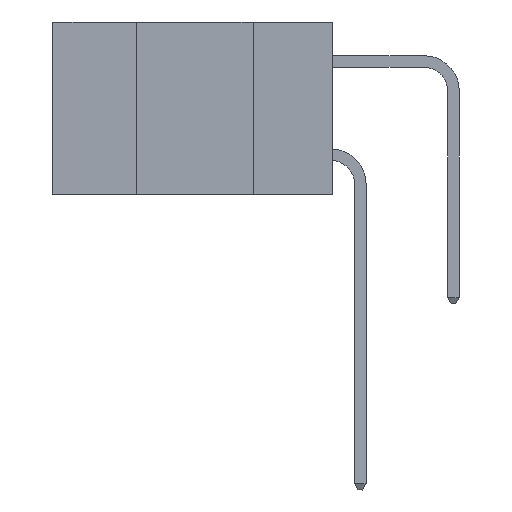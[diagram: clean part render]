
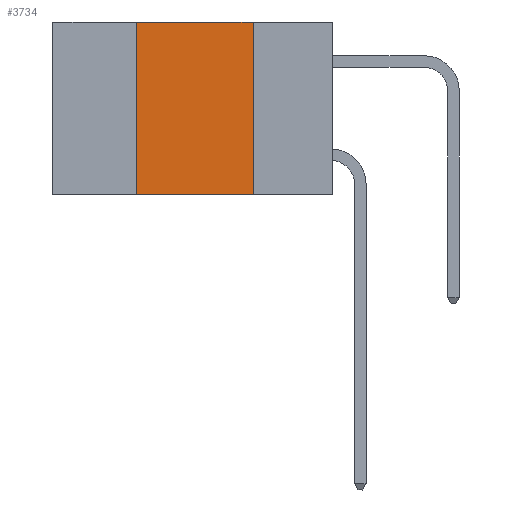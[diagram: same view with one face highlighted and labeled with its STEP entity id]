
A CAD part, left-side view. The second image highlights one B-rep face of the part: STEP entity #3734.
In plain terms, the highlighted planar face has unit normal (-1, 0, 0).
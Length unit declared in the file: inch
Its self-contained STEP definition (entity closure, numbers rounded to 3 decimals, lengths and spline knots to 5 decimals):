
#967 = EDGE_LOOP ( 'NONE', ( #6761, #6715, #1162, #23691 ) ) ;
#1009 = EDGE_CURVE ( 'NONE', #8339, #14403, #14055, .T. ) ;
#1162 = ORIENTED_EDGE ( 'NONE', *, *, #10354, .F. ) ;
#1880 = VERTEX_POINT ( 'NONE', #25369 ) ;
#2303 = FACE_OUTER_BOUND ( 'NONE', #967, .T. ) ;
#3734 = ADVANCED_FACE ( 'NONE', ( #2303 ), #18796, .F. ) ;
#4144 = VECTOR ( 'NONE', #8429, 39.37008 ) ;
#6715 = ORIENTED_EDGE ( 'NONE', *, *, #18160, .F. ) ;
#6761 = ORIENTED_EDGE ( 'NONE', *, *, #12855, .F. ) ;
#7384 = VECTOR ( 'NONE', #17304, 39.37008 ) ;
#8339 = VERTEX_POINT ( 'NONE', #14176 ) ;
#8429 = DIRECTION ( 'NONE',  ( 0., -1., 0. ) ) ;
#9397 = CARTESIAN_POINT ( 'NONE',  ( 0., 0.17, 0. ) ) ;
#10354 = EDGE_CURVE ( 'NONE', #8339, #1880, #13442, .T. ) ;
#10669 = LINE ( 'NONE', #15064, #16046 ) ;
#11346 = DIRECTION ( 'NONE',  ( 0., 0., -1. ) ) ;
#11915 = LINE ( 'NONE', #18263, #29262 ) ;
#12449 = DIRECTION ( 'NONE',  ( 0., 0., -1. ) ) ;
#12675 = DIRECTION ( 'NONE',  ( 1., 0., 0. ) ) ;
#12855 = EDGE_CURVE ( 'NONE', #19996, #14403, #11915, .T. ) ;
#13442 = LINE ( 'NONE', #24037, #7384 ) ;
#14055 = LINE ( 'NONE', #14223, #4144 ) ;
#14176 = CARTESIAN_POINT ( 'NONE',  ( 0., 0.42, -0.37 ) ) ;
#14223 = CARTESIAN_POINT ( 'NONE',  ( 0., 0.6, -0.37 ) ) ;
#14358 = CARTESIAN_POINT ( 'NONE',  ( 0., 0.17, -0.37 ) ) ;
#14403 = VERTEX_POINT ( 'NONE', #14358 ) ;
#15064 = CARTESIAN_POINT ( 'NONE',  ( 0., 0.6, 0. ) ) ;
#16046 = VECTOR ( 'NONE', #17374, 39.37008 ) ;
#17304 = DIRECTION ( 'NONE',  ( 0., 0., 1. ) ) ;
#17374 = DIRECTION ( 'NONE',  ( 0., -1., 0. ) ) ;
#18160 = EDGE_CURVE ( 'NONE', #1880, #19996, #10669, .T. ) ;
#18263 = CARTESIAN_POINT ( 'NONE',  ( 0., 0.17, 0. ) ) ;
#18796 = PLANE ( 'NONE',  #20945 ) ;
#19196 = CARTESIAN_POINT ( 'NONE',  ( 0., 0.6, 0. ) ) ;
#19996 = VERTEX_POINT ( 'NONE', #9397 ) ;
#20945 = AXIS2_PLACEMENT_3D ( 'NONE', #19196, #12675, #12449 ) ;
#23691 = ORIENTED_EDGE ( 'NONE', *, *, #1009, .T. ) ;
#24037 = CARTESIAN_POINT ( 'NONE',  ( 0., 0.42, 0. ) ) ;
#25369 = CARTESIAN_POINT ( 'NONE',  ( 0., 0.42, 0. ) ) ;
#29262 = VECTOR ( 'NONE', #11346, 39.37008 ) ;
